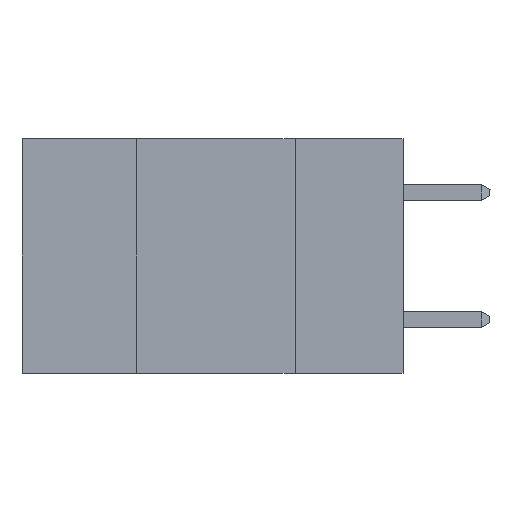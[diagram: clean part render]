
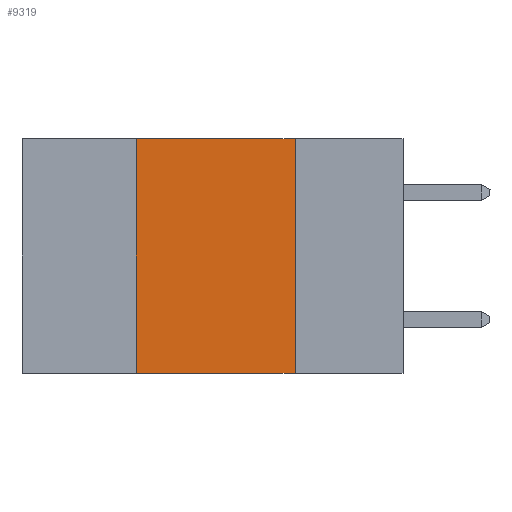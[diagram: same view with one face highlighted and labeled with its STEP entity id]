
A CAD part, left-side view. The second image highlights one B-rep face of the part: STEP entity #9319.
In plain terms, the highlighted planar face has unit normal (-1, 0, 0).
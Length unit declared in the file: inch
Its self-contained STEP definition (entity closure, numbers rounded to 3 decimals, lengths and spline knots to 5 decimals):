
#61 = PLANE ( 'NONE',  #1430 ) ;
#435 = DIRECTION ( 'NONE',  ( 0., -1., 0. ) ) ;
#788 = FACE_OUTER_BOUND ( 'NONE', #11676, .T. ) ;
#863 = CARTESIAN_POINT ( 'NONE',  ( 0., 0.17, 0. ) ) ;
#1329 = LINE ( 'NONE', #7329, #5611 ) ;
#1430 = AXIS2_PLACEMENT_3D ( 'NONE', #2979, #9777, #3943 ) ;
#2380 = VERTEX_POINT ( 'NONE', #863 ) ;
#2485 = DIRECTION ( 'NONE',  ( 0., 0., 1. ) ) ;
#2909 = LINE ( 'NONE', #3893, #7755 ) ;
#2933 = DIRECTION ( 'NONE',  ( 0., -1., 0. ) ) ;
#2979 = CARTESIAN_POINT ( 'NONE',  ( 0., 0.6, 0. ) ) ;
#3192 = EDGE_CURVE ( 'NONE', #2380, #8722, #7057, .T. ) ;
#3331 = ORIENTED_EDGE ( 'NONE', *, *, #3192, .F. ) ;
#3893 = CARTESIAN_POINT ( 'NONE',  ( 0., 0.6, 0. ) ) ;
#3943 = DIRECTION ( 'NONE',  ( 0., 0., -1. ) ) ;
#4278 = VECTOR ( 'NONE', #435, 39.37008 ) ;
#4580 = ORIENTED_EDGE ( 'NONE', *, *, #5915, .F. ) ;
#4590 = LINE ( 'NONE', #5273, #4278 ) ;
#5273 = CARTESIAN_POINT ( 'NONE',  ( 0., 0.6, -0.37 ) ) ;
#5611 = VECTOR ( 'NONE', #2485, 39.37008 ) ;
#5850 = CARTESIAN_POINT ( 'NONE',  ( 0., 0.17, 0. ) ) ;
#5915 = EDGE_CURVE ( 'NONE', #8474, #2380, #2909, .T. ) ;
#7057 = LINE ( 'NONE', #5850, #9345 ) ;
#7329 = CARTESIAN_POINT ( 'NONE',  ( 0., 0.42, 0. ) ) ;
#7603 = CARTESIAN_POINT ( 'NONE',  ( 0., 0.17, -0.37 ) ) ;
#7755 = VECTOR ( 'NONE', #2933, 39.37008 ) ;
#7935 = DIRECTION ( 'NONE',  ( 0., 0., -1. ) ) ;
#8474 = VERTEX_POINT ( 'NONE', #10001 ) ;
#8502 = EDGE_CURVE ( 'NONE', #12251, #8722, #4590, .T. ) ;
#8722 = VERTEX_POINT ( 'NONE', #7603 ) ;
#9319 = ADVANCED_FACE ( 'NONE', ( #788 ), #61, .F. ) ;
#9345 = VECTOR ( 'NONE', #7935, 39.37008 ) ;
#9777 = DIRECTION ( 'NONE',  ( 1., 0., 0. ) ) ;
#9892 = ORIENTED_EDGE ( 'NONE', *, *, #11592, .F. ) ;
#10001 = CARTESIAN_POINT ( 'NONE',  ( 0., 0.42, 0. ) ) ;
#11244 = CARTESIAN_POINT ( 'NONE',  ( 0., 0.42, -0.37 ) ) ;
#11518 = ORIENTED_EDGE ( 'NONE', *, *, #8502, .T. ) ;
#11592 = EDGE_CURVE ( 'NONE', #12251, #8474, #1329, .T. ) ;
#11676 = EDGE_LOOP ( 'NONE', ( #3331, #4580, #9892, #11518 ) ) ;
#12251 = VERTEX_POINT ( 'NONE', #11244 ) ;
